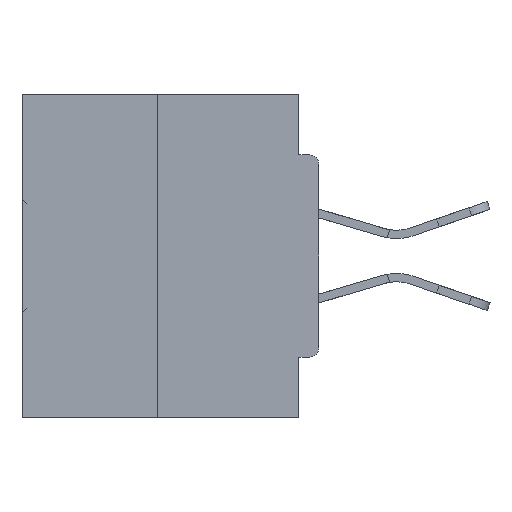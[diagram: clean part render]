
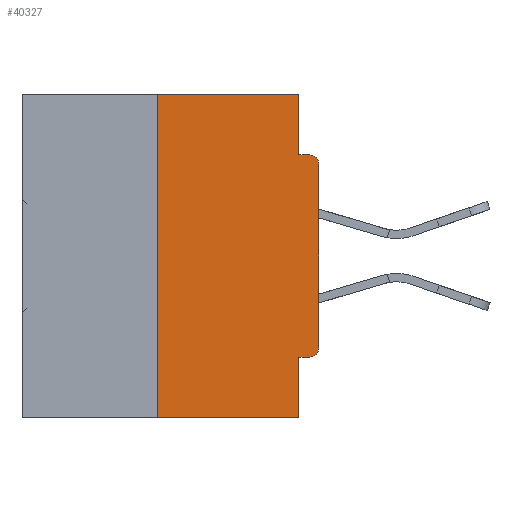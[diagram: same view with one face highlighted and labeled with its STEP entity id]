
A CAD part, left-side view. The second image highlights one B-rep face of the part: STEP entity #40327.
In plain terms, the highlighted planar face has unit normal (-1, 0, 0).
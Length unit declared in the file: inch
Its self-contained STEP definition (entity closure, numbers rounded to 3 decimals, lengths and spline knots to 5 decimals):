
#242 = CARTESIAN_POINT ( 'NONE',  ( 0., 0.031, -0.4065 ) ) ;
#1373 = VECTOR ( 'NONE', #25129, 39.37008 ) ;
#1954 = DIRECTION ( 'NONE',  ( 0., 0., -1. ) ) ;
#2588 = LINE ( 'NONE', #35094, #42086 ) ;
#3312 = CARTESIAN_POINT ( 'NONE',  ( 0., 0., -0.3915 ) ) ;
#3560 = VERTEX_POINT ( 'NONE', #10130 ) ;
#3570 = AXIS2_PLACEMENT_3D ( 'NONE', #44575, #26470, #1954 ) ;
#4209 = DIRECTION ( 'NONE',  ( 0., 0., -1. ) ) ;
#6168 = LINE ( 'NONE', #20540, #13420 ) ;
#6185 = ORIENTED_EDGE ( 'NONE', *, *, #8384, .F. ) ;
#8384 = EDGE_CURVE ( 'NONE', #22108, #41308, #12428, .T. ) ;
#8530 = ORIENTED_EDGE ( 'NONE', *, *, #32254, .T. ) ;
#8748 = DIRECTION ( 'NONE',  ( 0., 0., 1. ) ) ;
#9122 = ORIENTED_EDGE ( 'NONE', *, *, #23222, .T. ) ;
#9243 = CARTESIAN_POINT ( 'NONE',  ( 0., 0., -0.4065 ) ) ;
#10130 = CARTESIAN_POINT ( 'NONE',  ( 0., 0.031, 0. ) ) ;
#10220 = CIRCLE ( 'NONE', #29816, 0.015 ) ;
#10803 = EDGE_CURVE ( 'NONE', #43308, #11949, #45027, .T. ) ;
#11492 = DIRECTION ( 'NONE',  ( 1., 0., 0. ) ) ;
#11949 = VERTEX_POINT ( 'NONE', #242 ) ;
#12205 = CARTESIAN_POINT ( 'NONE',  ( 0., 0., -0.0935 ) ) ;
#12256 = ORIENTED_EDGE ( 'NONE', *, *, #40751, .T. ) ;
#12428 = LINE ( 'NONE', #12205, #14295 ) ;
#13420 = VECTOR ( 'NONE', #34891, 39.37008 ) ;
#14295 = VECTOR ( 'NONE', #30578, 39.37008 ) ;
#14760 = LINE ( 'NONE', #43015, #1373 ) ;
#14918 = CARTESIAN_POINT ( 'NONE',  ( 0., 0.46, -0.5 ) ) ;
#15011 = CARTESIAN_POINT ( 'NONE',  ( 0., 0.015, -0.4065 ) ) ;
#15038 = FACE_OUTER_BOUND ( 'NONE', #45243, .T. ) ;
#15240 = VERTEX_POINT ( 'NONE', #21096 ) ;
#15258 = ORIENTED_EDGE ( 'NONE', *, *, #36331, .F. ) ;
#15983 = LINE ( 'NONE', #38701, #25403 ) ;
#16290 = CARTESIAN_POINT ( 'NONE',  ( 0., 0.015, -0.0935 ) ) ;
#16761 = VERTEX_POINT ( 'NONE', #22764 ) ;
#20258 = CARTESIAN_POINT ( 'NONE',  ( 0., 0.46, 0. ) ) ;
#20540 = CARTESIAN_POINT ( 'NONE',  ( 0., 0.031, 0. ) ) ;
#20699 = ORIENTED_EDGE ( 'NONE', *, *, #30680, .T. ) ;
#20788 = ORIENTED_EDGE ( 'NONE', *, *, #22895, .F. ) ;
#21096 = CARTESIAN_POINT ( 'NONE',  ( 0., 0.031, -0.5 ) ) ;
#22108 = VERTEX_POINT ( 'NONE', #23466 ) ;
#22112 = CARTESIAN_POINT ( 'NONE',  ( 0., 0.015, -0.3915 ) ) ;
#22764 = CARTESIAN_POINT ( 'NONE',  ( 0., 0.25, -0.5 ) ) ;
#22895 = EDGE_CURVE ( 'NONE', #16761, #29403, #15983, .T. ) ;
#23222 = EDGE_CURVE ( 'NONE', #30826, #41308, #23890, .T. ) ;
#23466 = CARTESIAN_POINT ( 'NONE',  ( 0., 0.031, -0.0935 ) ) ;
#23484 = VERTEX_POINT ( 'NONE', #3312 ) ;
#23599 = DIRECTION ( 'NONE',  ( 0., 1., 0. ) ) ;
#23890 = CIRCLE ( 'NONE', #3570, 0.015 ) ;
#25129 = DIRECTION ( 'NONE',  ( 0., 0., -1. ) ) ;
#25403 = VECTOR ( 'NONE', #42457, 39.37008 ) ;
#25867 = DIRECTION ( 'NONE',  ( 0., 0., -1. ) ) ;
#26146 = VECTOR ( 'NONE', #23599, 39.37008 ) ;
#26470 = DIRECTION ( 'NONE',  ( -1., 0., 0. ) ) ;
#27447 = VECTOR ( 'NONE', #36339, 39.37008 ) ;
#27998 = LINE ( 'NONE', #20258, #33456 ) ;
#29105 = EDGE_CURVE ( 'NONE', #3560, #22108, #6168, .T. ) ;
#29403 = VERTEX_POINT ( 'NONE', #41665 ) ;
#29407 = PLANE ( 'NONE',  #31181 ) ;
#29816 = AXIS2_PLACEMENT_3D ( 'NONE', #22112, #36470, #4209 ) ;
#30578 = DIRECTION ( 'NONE',  ( 0., -1., 0. ) ) ;
#30680 = EDGE_CURVE ( 'NONE', #23484, #30826, #2588, .T. ) ;
#30826 = VERTEX_POINT ( 'NONE', #40986 ) ;
#31181 = AXIS2_PLACEMENT_3D ( 'NONE', #43747, #11492, #25867 ) ;
#32254 = EDGE_CURVE ( 'NONE', #43308, #23484, #10220, .T. ) ;
#33456 = VECTOR ( 'NONE', #34620, 39.37008 ) ;
#34620 = DIRECTION ( 'NONE',  ( 0., -1., 0. ) ) ;
#34891 = DIRECTION ( 'NONE',  ( 0., 0., -1. ) ) ;
#35094 = CARTESIAN_POINT ( 'NONE',  ( 0., 0., 0. ) ) ;
#36331 = EDGE_CURVE ( 'NONE', #11949, #15240, #14760, .T. ) ;
#36339 = DIRECTION ( 'NONE',  ( 0., -1., 0. ) ) ;
#36470 = DIRECTION ( 'NONE',  ( -1., 0., 0. ) ) ;
#38701 = CARTESIAN_POINT ( 'NONE',  ( 0., 0.25, 0. ) ) ;
#38743 = ORIENTED_EDGE ( 'NONE', *, *, #40146, .F. ) ;
#38773 = ORIENTED_EDGE ( 'NONE', *, *, #10803, .F. ) ;
#40146 = EDGE_CURVE ( 'NONE', #29403, #3560, #27998, .T. ) ;
#40327 = ADVANCED_FACE ( 'NONE', ( #15038 ), #29407, .F. ) ;
#40751 = EDGE_CURVE ( 'NONE', #16761, #15240, #43633, .T. ) ;
#40986 = CARTESIAN_POINT ( 'NONE',  ( 0., 0., -0.1085 ) ) ;
#41308 = VERTEX_POINT ( 'NONE', #16290 ) ;
#41665 = CARTESIAN_POINT ( 'NONE',  ( 0., 0.25, 0. ) ) ;
#42086 = VECTOR ( 'NONE', #8748, 39.37008 ) ;
#42457 = DIRECTION ( 'NONE',  ( 0., 0., 1. ) ) ;
#42572 = ORIENTED_EDGE ( 'NONE', *, *, #29105, .F. ) ;
#43015 = CARTESIAN_POINT ( 'NONE',  ( 0., 0.031, -0.5 ) ) ;
#43308 = VERTEX_POINT ( 'NONE', #15011 ) ;
#43633 = LINE ( 'NONE', #14918, #27447 ) ;
#43747 = CARTESIAN_POINT ( 'NONE',  ( 0., 0.46, 0. ) ) ;
#44575 = CARTESIAN_POINT ( 'NONE',  ( 0., 0.015, -0.1085 ) ) ;
#45027 = LINE ( 'NONE', #9243, #26146 ) ;
#45243 = EDGE_LOOP ( 'NONE', ( #38743, #20788, #12256, #15258, #38773, #8530, #20699, #9122, #6185, #42572 ) ) ;
